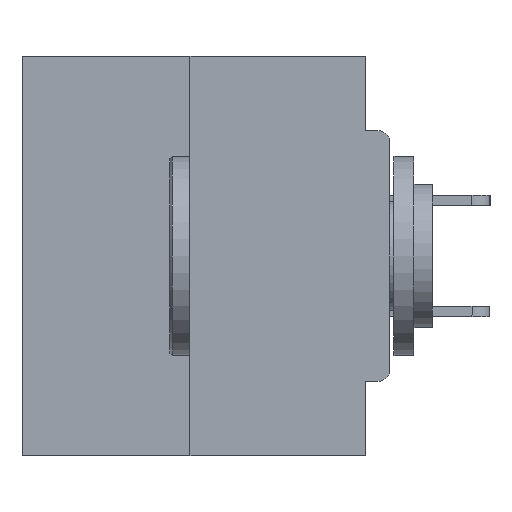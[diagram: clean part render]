
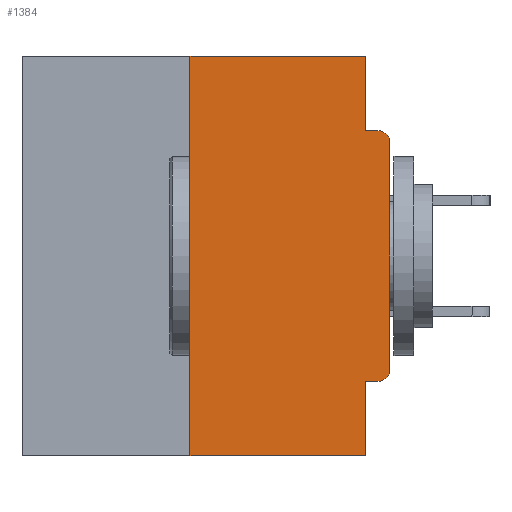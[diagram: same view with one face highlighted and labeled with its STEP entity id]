
A CAD part, left-side view. The second image highlights one B-rep face of the part: STEP entity #1384.
In plain terms, the highlighted planar face has unit normal (-1, 0, 0).
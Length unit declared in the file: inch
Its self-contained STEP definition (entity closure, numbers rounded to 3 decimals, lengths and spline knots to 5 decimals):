
#130 = ORIENTED_EDGE ( 'NONE', *, *, #3981, .F. ) ;
#566 = EDGE_CURVE ( 'NONE', #32287, #14350, #26810, .T. ) ;
#1196 = LINE ( 'NONE', #39809, #25297 ) ;
#1384 = ADVANCED_FACE ( 'NONE', ( #10918 ), #15258, .F. ) ;
#1545 = DIRECTION ( 'NONE',  ( 0., -1., 0. ) ) ;
#2383 = VERTEX_POINT ( 'NONE', #14359 ) ;
#2487 = DIRECTION ( 'NONE',  ( 0., 0., -1. ) ) ;
#2673 = DIRECTION ( 'NONE',  ( 0., 0., -1. ) ) ;
#2987 = DIRECTION ( 'NONE',  ( 0., 0., 1. ) ) ;
#3027 = EDGE_CURVE ( 'NONE', #13043, #36866, #11285, .T. ) ;
#3981 = EDGE_CURVE ( 'NONE', #4904, #32287, #28483, .T. ) ;
#4016 = ORIENTED_EDGE ( 'NONE', *, *, #3027, .T. ) ;
#4258 = EDGE_LOOP ( 'NONE', ( #38144, #30267, #29541, #28423, #11599, #33065, #4016, #22356, #13373, #130 ) ) ;
#4904 = VERTEX_POINT ( 'NONE', #8117 ) ;
#5240 = DIRECTION ( 'NONE',  ( 1., 0., 0. ) ) ;
#6609 = CARTESIAN_POINT ( 'NONE',  ( 0., 0.015, -0.0935 ) ) ;
#8117 = CARTESIAN_POINT ( 'NONE',  ( 0., 0.031, 0. ) ) ;
#8450 = VECTOR ( 'NONE', #34445, 39.37008 ) ;
#9062 = VECTOR ( 'NONE', #1545, 39.37008 ) ;
#9074 = VECTOR ( 'NONE', #21664, 39.37008 ) ;
#9198 = VERTEX_POINT ( 'NONE', #28217 ) ;
#9346 = CARTESIAN_POINT ( 'NONE',  ( 0., 0.031, -0.0935 ) ) ;
#10031 = EDGE_CURVE ( 'NONE', #11064, #11036, #10581, .T. ) ;
#10581 = LINE ( 'NONE', #15347, #9074 ) ;
#10918 = FACE_OUTER_BOUND ( 'NONE', #4258, .T. ) ;
#11036 = VERTEX_POINT ( 'NONE', #30723 ) ;
#11064 = VERTEX_POINT ( 'NONE', #27722 ) ;
#11285 = LINE ( 'NONE', #21677, #40278 ) ;
#11599 = ORIENTED_EDGE ( 'NONE', *, *, #22826, .F. ) ;
#11890 = VECTOR ( 'NONE', #28859, 39.37008 ) ;
#12966 = CARTESIAN_POINT ( 'NONE',  ( 0., 0.46, 0. ) ) ;
#13043 = VERTEX_POINT ( 'NONE', #27187 ) ;
#13368 = EDGE_CURVE ( 'NONE', #11036, #4904, #21760, .T. ) ;
#13373 = ORIENTED_EDGE ( 'NONE', *, *, #566, .F. ) ;
#14350 = VERTEX_POINT ( 'NONE', #6609 ) ;
#14359 = CARTESIAN_POINT ( 'NONE',  ( 0., 0.031, -0.4065 ) ) ;
#15258 = PLANE ( 'NONE',  #33351 ) ;
#15347 = CARTESIAN_POINT ( 'NONE',  ( 0., 0.25, 0. ) ) ;
#17821 = DIRECTION ( 'NONE',  ( 0., 0., -1. ) ) ;
#18426 = CARTESIAN_POINT ( 'NONE',  ( 0., 0.46, 0. ) ) ;
#19648 = CARTESIAN_POINT ( 'NONE',  ( 0., 0.031, -0.5 ) ) ;
#20237 = EDGE_CURVE ( 'NONE', #9198, #13043, #39590, .T. ) ;
#21664 = DIRECTION ( 'NONE',  ( 0., 0., 1. ) ) ;
#21677 = CARTESIAN_POINT ( 'NONE',  ( 0., 0., 0. ) ) ;
#21712 = DIRECTION ( 'NONE',  ( 0., 0., -1. ) ) ;
#21760 = LINE ( 'NONE', #12966, #8450 ) ;
#22264 = LINE ( 'NONE', #34371, #28219 ) ;
#22356 = ORIENTED_EDGE ( 'NONE', *, *, #24692, .T. ) ;
#22826 = EDGE_CURVE ( 'NONE', #9198, #2383, #31620, .T. ) ;
#22935 = AXIS2_PLACEMENT_3D ( 'NONE', #24820, #27873, #2673 ) ;
#23868 = VERTEX_POINT ( 'NONE', #19648 ) ;
#23914 = DIRECTION ( 'NONE',  ( 0., -1., 0. ) ) ;
#24150 = DIRECTION ( 'NONE',  ( -1., 0., 0. ) ) ;
#24692 = EDGE_CURVE ( 'NONE', #36866, #14350, #34924, .T. ) ;
#24820 = CARTESIAN_POINT ( 'NONE',  ( 0., 0.015, -0.1085 ) ) ;
#25297 = VECTOR ( 'NONE', #23914, 39.37008 ) ;
#26415 = CARTESIAN_POINT ( 'NONE',  ( 0., 0., -0.0935 ) ) ;
#26810 = LINE ( 'NONE', #26415, #9062 ) ;
#27187 = CARTESIAN_POINT ( 'NONE',  ( 0., 0., -0.3915 ) ) ;
#27722 = CARTESIAN_POINT ( 'NONE',  ( 0., 0.25, -0.5 ) ) ;
#27873 = DIRECTION ( 'NONE',  ( -1., 0., 0. ) ) ;
#27995 = VECTOR ( 'NONE', #37656, 39.37008 ) ;
#28217 = CARTESIAN_POINT ( 'NONE',  ( 0., 0.015, -0.4065 ) ) ;
#28219 = VECTOR ( 'NONE', #21712, 39.37008 ) ;
#28423 = ORIENTED_EDGE ( 'NONE', *, *, #34971, .F. ) ;
#28483 = LINE ( 'NONE', #28891, #27995 ) ;
#28560 = EDGE_CURVE ( 'NONE', #11064, #23868, #1196, .T. ) ;
#28859 = DIRECTION ( 'NONE',  ( 0., 1., 0. ) ) ;
#28891 = CARTESIAN_POINT ( 'NONE',  ( 0., 0.031, 0. ) ) ;
#29541 = ORIENTED_EDGE ( 'NONE', *, *, #28560, .T. ) ;
#30267 = ORIENTED_EDGE ( 'NONE', *, *, #10031, .F. ) ;
#30347 = CARTESIAN_POINT ( 'NONE',  ( 0., 0.015, -0.3915 ) ) ;
#30521 = CARTESIAN_POINT ( 'NONE',  ( 0., 0., -0.1085 ) ) ;
#30723 = CARTESIAN_POINT ( 'NONE',  ( 0., 0.25, 0. ) ) ;
#31620 = LINE ( 'NONE', #37754, #11890 ) ;
#32287 = VERTEX_POINT ( 'NONE', #9346 ) ;
#33065 = ORIENTED_EDGE ( 'NONE', *, *, #20237, .T. ) ;
#33351 = AXIS2_PLACEMENT_3D ( 'NONE', #18426, #5240, #2487 ) ;
#34161 = AXIS2_PLACEMENT_3D ( 'NONE', #30347, #24150, #17821 ) ;
#34371 = CARTESIAN_POINT ( 'NONE',  ( 0., 0.031, -0.5 ) ) ;
#34445 = DIRECTION ( 'NONE',  ( 0., -1., 0. ) ) ;
#34924 = CIRCLE ( 'NONE', #22935, 0.015 ) ;
#34971 = EDGE_CURVE ( 'NONE', #2383, #23868, #22264, .T. ) ;
#36866 = VERTEX_POINT ( 'NONE', #30521 ) ;
#37656 = DIRECTION ( 'NONE',  ( 0., 0., -1. ) ) ;
#37754 = CARTESIAN_POINT ( 'NONE',  ( 0., 0., -0.4065 ) ) ;
#38144 = ORIENTED_EDGE ( 'NONE', *, *, #13368, .F. ) ;
#39590 = CIRCLE ( 'NONE', #34161, 0.015 ) ;
#39809 = CARTESIAN_POINT ( 'NONE',  ( 0., 0.46, -0.5 ) ) ;
#40278 = VECTOR ( 'NONE', #2987, 39.37008 ) ;
